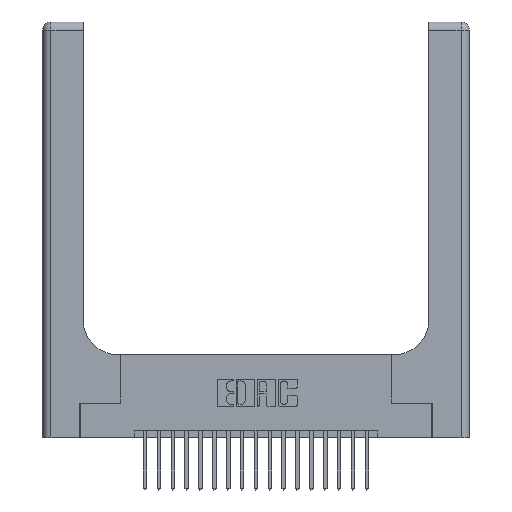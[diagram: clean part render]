
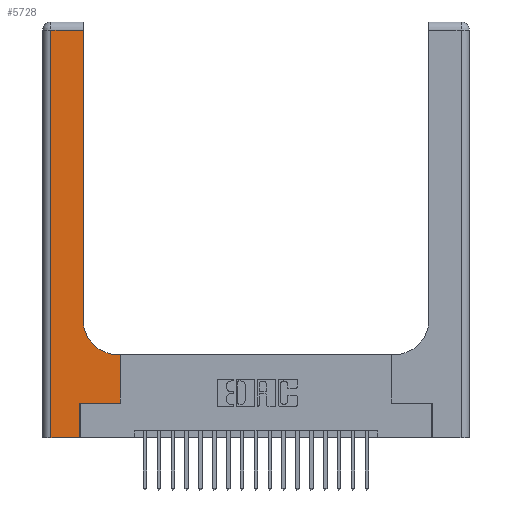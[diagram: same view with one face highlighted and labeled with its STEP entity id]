
A CAD part, top view. The second image highlights one B-rep face of the part: STEP entity #5728.
In plain terms, the highlighted planar face has unit normal (0, 0, 1).
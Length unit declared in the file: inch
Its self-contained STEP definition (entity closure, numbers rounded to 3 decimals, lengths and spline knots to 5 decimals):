
#400 = LINE ( 'NONE', #10411, #9134 ) ;
#499 = CARTESIAN_POINT ( 'NONE',  ( 0.2915, 0.85, 0.37 ) ) ;
#504 = CARTESIAN_POINT ( 'NONE',  ( 0.2915, 2.94, 0.37 ) ) ;
#1336 = VECTOR ( 'NONE', #6965, 39.37008 ) ;
#1349 = VERTEX_POINT ( 'NONE', #6141 ) ;
#1423 = CARTESIAN_POINT ( 'NONE',  ( 0.5585, 0.25, 0.37 ) ) ;
#1697 = EDGE_CURVE ( 'NONE', #12777, #6527, #16525, .T. ) ;
#2390 = CARTESIAN_POINT ( 'NONE',  ( 0.2915, 3., 0.37 ) ) ;
#2397 = LINE ( 'NONE', #3290, #8236 ) ;
#2608 = ORIENTED_EDGE ( 'NONE', *, *, #14074, .T. ) ;
#2669 = DIRECTION ( 'NONE',  ( -1., 0., 0. ) ) ;
#2697 = DIRECTION ( 'NONE',  ( 0., 0., -1. ) ) ;
#2939 = CARTESIAN_POINT ( 'NONE',  ( 0.06, 0., 0.37 ) ) ;
#3290 = CARTESIAN_POINT ( 'NONE',  ( 0., 2.94, 0.37 ) ) ;
#3520 = ORIENTED_EDGE ( 'NONE', *, *, #6116, .T. ) ;
#4312 = CARTESIAN_POINT ( 'NONE',  ( 0.06, 3., 0.37 ) ) ;
#4382 = CARTESIAN_POINT ( 'NONE',  ( 0.2915, 0.6, 0.37 ) ) ;
#4397 = ORIENTED_EDGE ( 'NONE', *, *, #5845, .T. ) ;
#4428 = ORIENTED_EDGE ( 'NONE', *, *, #1697, .T. ) ;
#4924 = LINE ( 'NONE', #2390, #18158 ) ;
#5265 = ORIENTED_EDGE ( 'NONE', *, *, #5753, .T. ) ;
#5323 = VERTEX_POINT ( 'NONE', #1423 ) ;
#5498 = AXIS2_PLACEMENT_3D ( 'NONE', #9351, #2697, #21193 ) ;
#5728 = ADVANCED_FACE ( 'NONE', ( #11131 ), #18602, .F. ) ;
#5753 = EDGE_CURVE ( 'NONE', #11979, #1349, #2397, .T. ) ;
#5837 = LINE ( 'NONE', #12221, #1336 ) ;
#5845 = EDGE_CURVE ( 'NONE', #5323, #14458, #5837, .T. ) ;
#6116 = EDGE_CURVE ( 'NONE', #14458, #11722, #13755, .T. ) ;
#6141 = CARTESIAN_POINT ( 'NONE',  ( 0.06, 2.94, 0.37 ) ) ;
#6509 = VERTEX_POINT ( 'NONE', #499 ) ;
#6527 = VERTEX_POINT ( 'NONE', #12196 ) ;
#6570 = ORIENTED_EDGE ( 'NONE', *, *, #14637, .T. ) ;
#6710 = VECTOR ( 'NONE', #7845, 39.37008 ) ;
#6965 = DIRECTION ( 'NONE',  ( 0., 1., 0. ) ) ;
#7078 = EDGE_LOOP ( 'NONE', ( #20085, #5265, #6570, #4428, #2608, #13947, #4397, #3520, #17732 ) ) ;
#7293 = DIRECTION ( 'NONE',  ( 0., 1., 0. ) ) ;
#7845 = DIRECTION ( 'NONE',  ( 0., -1., 0. ) ) ;
#7864 = DIRECTION ( 'NONE',  ( -1., 0., 0. ) ) ;
#8236 = VECTOR ( 'NONE', #7864, 39.37008 ) ;
#8447 = DIRECTION ( 'NONE',  ( 0., 0., -1. ) ) ;
#8641 = DIRECTION ( 'NONE',  ( 0., 1., 0. ) ) ;
#9134 = VECTOR ( 'NONE', #8641, 39.37008 ) ;
#9351 = CARTESIAN_POINT ( 'NONE',  ( 0.5415, 0.85, 0.37 ) ) ;
#9373 = LINE ( 'NONE', #4312, #6710 ) ;
#10411 = CARTESIAN_POINT ( 'NONE',  ( 0.269, 0., 0.37 ) ) ;
#11045 = CARTESIAN_POINT ( 'NONE',  ( 0.269, 0.25, 0.37 ) ) ;
#11131 = FACE_OUTER_BOUND ( 'NONE', #7078, .T. ) ;
#11722 = VERTEX_POINT ( 'NONE', #13310 ) ;
#11979 = VERTEX_POINT ( 'NONE', #504 ) ;
#12196 = CARTESIAN_POINT ( 'NONE',  ( 0.269, 0., 0.37 ) ) ;
#12221 = CARTESIAN_POINT ( 'NONE',  ( 0.5585, 0.25, 0.37 ) ) ;
#12777 = VERTEX_POINT ( 'NONE', #2939 ) ;
#13063 = VECTOR ( 'NONE', #13643, 39.37008 ) ;
#13117 = VERTEX_POINT ( 'NONE', #14865 ) ;
#13259 = EDGE_CURVE ( 'NONE', #6509, #11979, #4924, .T. ) ;
#13310 = CARTESIAN_POINT ( 'NONE',  ( 0.5415, 0.6, 0.37 ) ) ;
#13434 = EDGE_CURVE ( 'NONE', #13117, #5323, #20294, .T. ) ;
#13542 = AXIS2_PLACEMENT_3D ( 'NONE', #16674, #8447, #21765 ) ;
#13643 = DIRECTION ( 'NONE',  ( 1., 0., 0. ) ) ;
#13755 = LINE ( 'NONE', #4382, #16945 ) ;
#13947 = ORIENTED_EDGE ( 'NONE', *, *, #13434, .T. ) ;
#14074 = EDGE_CURVE ( 'NONE', #6527, #13117, #400, .T. ) ;
#14458 = VERTEX_POINT ( 'NONE', #20872 ) ;
#14637 = EDGE_CURVE ( 'NONE', #1349, #12777, #9373, .T. ) ;
#14865 = CARTESIAN_POINT ( 'NONE',  ( 0.269, 0.25, 0.37 ) ) ;
#15211 = CARTESIAN_POINT ( 'NONE',  ( 0., 0., 0.37 ) ) ;
#15836 = CIRCLE ( 'NONE', #5498, 0.25 ) ;
#16525 = LINE ( 'NONE', #15211, #13063 ) ;
#16674 = CARTESIAN_POINT ( 'NONE',  ( 0., 3., 0.37 ) ) ;
#16945 = VECTOR ( 'NONE', #2669, 39.37008 ) ;
#17732 = ORIENTED_EDGE ( 'NONE', *, *, #20991, .T. ) ;
#18158 = VECTOR ( 'NONE', #7293, 39.37008 ) ;
#18602 = PLANE ( 'NONE',  #13542 ) ;
#19643 = DIRECTION ( 'NONE',  ( 1., 0., 0. ) ) ;
#20085 = ORIENTED_EDGE ( 'NONE', *, *, #13259, .T. ) ;
#20294 = LINE ( 'NONE', #11045, #21342 ) ;
#20872 = CARTESIAN_POINT ( 'NONE',  ( 0.5585, 0.6, 0.37 ) ) ;
#20991 = EDGE_CURVE ( 'NONE', #11722, #6509, #15836, .T. ) ;
#21193 = DIRECTION ( 'NONE',  ( 1., 0., 0. ) ) ;
#21342 = VECTOR ( 'NONE', #19643, 39.37008 ) ;
#21765 = DIRECTION ( 'NONE',  ( -1., 0., 0. ) ) ;
